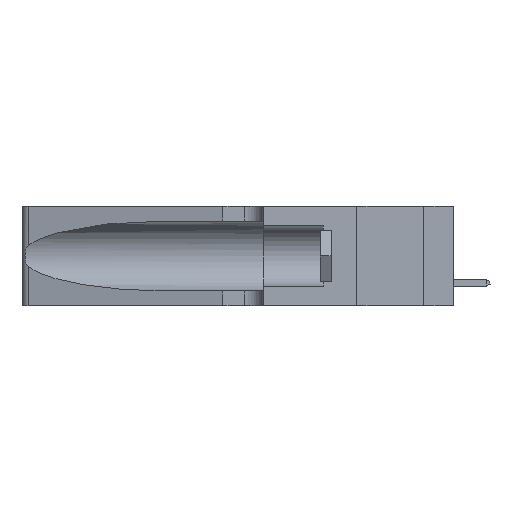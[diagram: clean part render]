
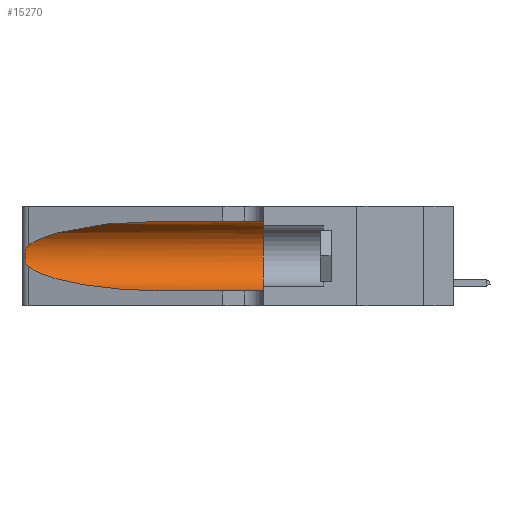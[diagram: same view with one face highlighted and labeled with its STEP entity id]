
A CAD part, left-side view. The second image highlights one B-rep face of the part: STEP entity #15270.
In plain terms, the highlighted cylindrical face has radius 3.308 mm (diameter 6.617 mm), a partial arc.
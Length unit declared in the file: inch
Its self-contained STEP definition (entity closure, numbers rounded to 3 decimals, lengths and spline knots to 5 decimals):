
#990 = CARTESIAN_POINT ( 'NONE',  ( 0.26018, 1.23835, 0.19895 ) ) ;
#1077 = VECTOR ( 'NONE', #21580, 39.37008 ) ;
#1100 =( BOUNDED_CURVE ( )  B_SPLINE_CURVE ( 3, ( #6994, #30394, #33838, #18991 ),
 .UNSPECIFIED., .F., .F. ) 
 B_SPLINE_CURVE_WITH_KNOTS ( ( 4, 4 ),
 ( 3.44316, 4.71239 ),
 .UNSPECIFIED. ) 
 CURVE ( )  GEOMETRIC_REPRESENTATION_ITEM ( )  RATIONAL_B_SPLINE_CURVE ( ( 1., 0.87, 0.87, 1. ) ) 
 REPRESENTATION_ITEM ( '' )  );
#1143 = DIRECTION ( 'NONE',  ( 0., -1., 0. ) ) ;
#1192 = CYLINDRICAL_SURFACE ( 'NONE', #15779, 0.13025 ) ;
#1218 = CARTESIAN_POINT ( 'NONE',  ( 0.1305, 0.35, 0.185 ) ) ;
#2876 = CARTESIAN_POINT ( 'NONE',  ( 0.25487, 1.22718, 0.22369 ) ) ;
#5675 =( BOUNDED_CURVE ( )  B_SPLINE_CURVE ( 3, ( #31795, #22633, #7925, #14092 ),
 .UNSPECIFIED., .F., .F. ) 
 B_SPLINE_CURVE_WITH_KNOTS ( ( 4, 4 ),
 ( 1.5708, 2.84003 ),
 .UNSPECIFIED. ) 
 CURVE ( )  GEOMETRIC_REPRESENTATION_ITEM ( )  RATIONAL_B_SPLINE_CURVE ( ( 1., 0.87, 0.87, 1. ) ) 
 REPRESENTATION_ITEM ( '' )  );
#6221 = CARTESIAN_POINT ( 'NONE',  ( 0.25487, 1.22718, 0.22369 ) ) ;
#6291 = CARTESIAN_POINT ( 'NONE',  ( 0.1305, 1.61858, 0.31525 ) ) ;
#6400 = CARTESIAN_POINT ( 'NONE',  ( 0.25487, 1.22718, 0.14631 ) ) ;
#6994 = CARTESIAN_POINT ( 'NONE',  ( 0.25487, 1.22718, 0.14631 ) ) ;
#7123 = EDGE_CURVE ( 'NONE', #21999, #20783, #5675, .T. ) ;
#7271 = VERTEX_POINT ( 'NONE', #13435 ) ;
#7925 = CARTESIAN_POINT ( 'NONE',  ( 0.2373, 1.15595, 0.28018 ) ) ;
#8807 = ORIENTED_EDGE ( 'NONE', *, *, #19509, .T. ) ;
#8825 = CARTESIAN_POINT ( 'NONE',  ( 0.25555, 1.22994, 0.2215 ) ) ;
#8956 = LINE ( 'NONE', #30370, #1077 ) ;
#10048 = CARTESIAN_POINT ( 'NONE',  ( 0.26017, 1.23833, 0.17102 ) ) ;
#10253 = DIRECTION ( 'NONE',  ( 0., 0., 1. ) ) ;
#10306 = CARTESIAN_POINT ( 'NONE',  ( 0.25555, 1.22993, 0.14849 ) ) ;
#10323 = DIRECTION ( 'NONE',  ( 0., 0., -1. ) ) ;
#11211 = EDGE_LOOP ( 'NONE', ( #26448, #33962, #34361, #8807, #11247, #36106 ) ) ;
#11247 = ORIENTED_EDGE ( 'NONE', *, *, #28684, .F. ) ;
#12016 = CARTESIAN_POINT ( 'NONE',  ( 0.25787, 1.23484, 0.2124 ) ) ;
#12869 = CARTESIAN_POINT ( 'NONE',  ( 0.26075, 1.23896, 0.178 ) ) ;
#13079 = DIRECTION ( 'NONE',  ( 0., 1., 0. ) ) ;
#13268 = CARTESIAN_POINT ( 'NONE',  ( 0.26075, 1.23896, 0.19203 ) ) ;
#13435 = CARTESIAN_POINT ( 'NONE',  ( 0.1305, 0.35, 0.05475 ) ) ;
#14092 = CARTESIAN_POINT ( 'NONE',  ( 0.25487, 1.22718, 0.22369 ) ) ;
#14132 = VERTEX_POINT ( 'NONE', #17029 ) ;
#15270 = ADVANCED_FACE ( 'NONE', ( #28982 ), #1192, .F. ) ;
#15779 = AXIS2_PLACEMENT_3D ( 'NONE', #25341, #1143, #10323 ) ;
#16655 = LINE ( 'NONE', #6291, #31006 ) ;
#17029 = CARTESIAN_POINT ( 'NONE',  ( 0.1305, 0.35, 0.31525 ) ) ;
#18991 = CARTESIAN_POINT ( 'NONE',  ( 0.1305, 0.72297, 0.05475 ) ) ;
#19509 = EDGE_CURVE ( 'NONE', #37272, #7271, #8956, .T. ) ;
#20783 = VERTEX_POINT ( 'NONE', #6221 ) ;
#21138 = DIRECTION ( 'NONE',  ( 0., -1., 0. ) ) ;
#21201 = EDGE_CURVE ( 'NONE', #21999, #14132, #16655, .T. ) ;
#21580 = DIRECTION ( 'NONE',  ( 0., -1., 0. ) ) ;
#21999 = VERTEX_POINT ( 'NONE', #30866 ) ;
#22195 = CARTESIAN_POINT ( 'NONE',  ( 0.25856, 1.23593, 0.16098 ) ) ;
#22633 = CARTESIAN_POINT ( 'NONE',  ( 0.18966, 0.96281, 0.31525 ) ) ;
#24223 = EDGE_CURVE ( 'NONE', #35353, #37272, #1100, .T. ) ;
#24646 = CARTESIAN_POINT ( 'NONE',  ( 0.25487, 1.22718, 0.14631 ) ) ;
#25190 = CARTESIAN_POINT ( 'NONE',  ( 0.25639, 1.23186, 0.15144 ) ) ;
#25341 = CARTESIAN_POINT ( 'NONE',  ( 0.1305, 1.61858, 0.185 ) ) ;
#26448 = ORIENTED_EDGE ( 'NONE', *, *, #7123, .T. ) ;
#27899 = CARTESIAN_POINT ( 'NONE',  ( 0.25854, 1.2359, 0.20912 ) ) ;
#28684 = EDGE_CURVE ( 'NONE', #14132, #7271, #32625, .T. ) ;
#28982 = FACE_OUTER_BOUND ( 'NONE', #11211, .T. ) ;
#29701 = AXIS2_PLACEMENT_3D ( 'NONE', #1218, #13079, #10253 ) ;
#29739 = CARTESIAN_POINT ( 'NONE',  ( 0.25639, 1.23184, 0.21858 ) ) ;
#30370 = CARTESIAN_POINT ( 'NONE',  ( 0.1305, 1.61858, 0.05475 ) ) ;
#30394 = CARTESIAN_POINT ( 'NONE',  ( 0.2373, 1.15595, 0.08982 ) ) ;
#30866 = CARTESIAN_POINT ( 'NONE',  ( 0.1305, 0.72297, 0.31525 ) ) ;
#31006 = VECTOR ( 'NONE', #21138, 39.37008 ) ;
#31795 = CARTESIAN_POINT ( 'NONE',  ( 0.1305, 0.72297, 0.31525 ) ) ;
#32625 = CIRCLE ( 'NONE', #29701, 0.13025 ) ;
#33838 = CARTESIAN_POINT ( 'NONE',  ( 0.18966, 0.96281, 0.05475 ) ) ;
#33962 = ORIENTED_EDGE ( 'NONE', *, *, #37776, .T. ) ;
#34361 = ORIENTED_EDGE ( 'NONE', *, *, #24223, .T. ) ;
#34757 = B_SPLINE_CURVE_WITH_KNOTS ( 'NONE', 3,
 ( #2876, #8825, #29739, #12016, #27899, #990, #13268, #12869, #10048, #22195, #36903, #25190, #10306, #24646 ),
 .UNSPECIFIED., .F., .F.,
 ( 4, 2, 2, 2, 2, 2, 4 ),
 ( 0., 0.00027, 0.00053, 0.00107, 0.0016, 0.00187, 0.00214 ),
 .UNSPECIFIED. ) ;
#35353 = VERTEX_POINT ( 'NONE', #6400 ) ;
#36106 = ORIENTED_EDGE ( 'NONE', *, *, #21201, .F. ) ;
#36588 = CARTESIAN_POINT ( 'NONE',  ( 0.1305, 0.72297, 0.05475 ) ) ;
#36903 = CARTESIAN_POINT ( 'NONE',  ( 0.25789, 1.23486, 0.15765 ) ) ;
#37272 = VERTEX_POINT ( 'NONE', #36588 ) ;
#37776 = EDGE_CURVE ( 'NONE', #20783, #35353, #34757, .T. ) ;
